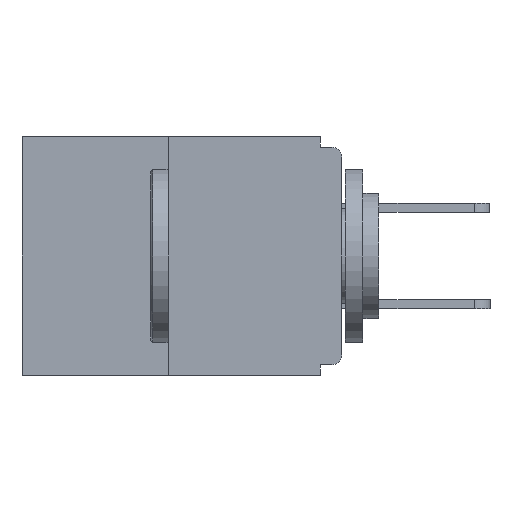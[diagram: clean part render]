
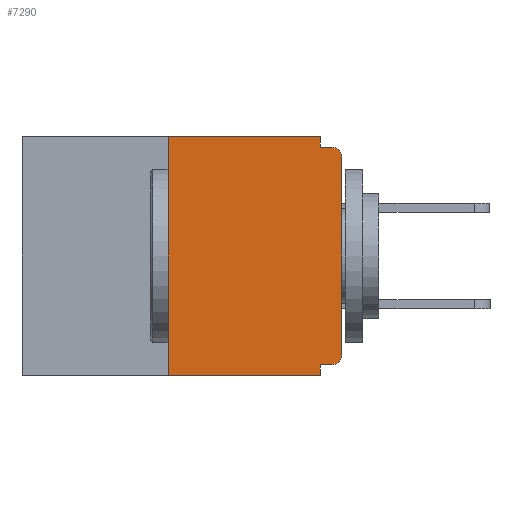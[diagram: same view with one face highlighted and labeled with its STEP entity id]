
A CAD part, left-side view. The second image highlights one B-rep face of the part: STEP entity #7290.
In plain terms, the highlighted planar face has unit normal (-1, 0, 0).
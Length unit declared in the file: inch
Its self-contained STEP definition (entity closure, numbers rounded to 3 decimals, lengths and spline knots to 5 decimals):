
#361 = DIRECTION ( 'NONE',  ( 1., 0., 0. ) ) ;
#381 = CARTESIAN_POINT ( 'NONE',  ( 0., 0.015, -0.03 ) ) ;
#546 = DIRECTION ( 'NONE',  ( 0., 0., -1. ) ) ;
#837 = CARTESIAN_POINT ( 'NONE',  ( 0., 0.25, 0. ) ) ;
#869 = CARTESIAN_POINT ( 'NONE',  ( 0., 0., 0. ) ) ;
#1276 = DIRECTION ( 'NONE',  ( 0., 0., -1. ) ) ;
#1318 = VECTOR ( 'NONE', #1604, 39.37008 ) ;
#1597 = CARTESIAN_POINT ( 'NONE',  ( 0., 0., -0.03 ) ) ;
#1604 = DIRECTION ( 'NONE',  ( 0., 0., -1. ) ) ;
#1741 = CARTESIAN_POINT ( 'NONE',  ( 0., 0., -0.313 ) ) ;
#1835 = CIRCLE ( 'NONE', #3360, 0.015 ) ;
#1837 = CARTESIAN_POINT ( 'NONE',  ( 0., 0.46, 0. ) ) ;
#1895 = CARTESIAN_POINT ( 'NONE',  ( 0., 0.25, 0. ) ) ;
#2158 = CARTESIAN_POINT ( 'NONE',  ( 0., 0.46, -0.343 ) ) ;
#2202 = LINE ( 'NONE', #4541, #16559 ) ;
#2294 = CARTESIAN_POINT ( 'NONE',  ( 0., 0., -0.328 ) ) ;
#2396 = ORIENTED_EDGE ( 'NONE', *, *, #13803, .T. ) ;
#2406 = DIRECTION ( 'NONE',  ( 0., 0., 1. ) ) ;
#3265 = VERTEX_POINT ( 'NONE', #7726 ) ;
#3360 = AXIS2_PLACEMENT_3D ( 'NONE', #381, #18469, #16746 ) ;
#4233 = ORIENTED_EDGE ( 'NONE', *, *, #10273, .T. ) ;
#4315 = CARTESIAN_POINT ( 'NONE',  ( 0., 0.031, -0.328 ) ) ;
#4493 = ORIENTED_EDGE ( 'NONE', *, *, #6026, .F. ) ;
#4526 = VERTEX_POINT ( 'NONE', #5584 ) ;
#4541 = CARTESIAN_POINT ( 'NONE',  ( 0., 0., -0.015 ) ) ;
#4764 = VERTEX_POINT ( 'NONE', #16749 ) ;
#5029 = ORIENTED_EDGE ( 'NONE', *, *, #14494, .F. ) ;
#5207 = EDGE_CURVE ( 'NONE', #5364, #18720, #5545, .T. ) ;
#5218 = ORIENTED_EDGE ( 'NONE', *, *, #16692, .F. ) ;
#5275 = VECTOR ( 'NONE', #16773, 39.37008 ) ;
#5364 = VERTEX_POINT ( 'NONE', #1741 ) ;
#5411 = VECTOR ( 'NONE', #18132, 39.37008 ) ;
#5515 = AXIS2_PLACEMENT_3D ( 'NONE', #13824, #361, #546 ) ;
#5545 = LINE ( 'NONE', #869, #19473 ) ;
#5584 = CARTESIAN_POINT ( 'NONE',  ( 0., 0.015, -0.015 ) ) ;
#5705 = ORIENTED_EDGE ( 'NONE', *, *, #17068, .F. ) ;
#5781 = LINE ( 'NONE', #8175, #14447 ) ;
#5806 = DIRECTION ( 'NONE',  ( -1., 0., 0. ) ) ;
#6026 = EDGE_CURVE ( 'NONE', #11294, #4526, #2202, .T. ) ;
#6120 = CARTESIAN_POINT ( 'NONE',  ( 0., 0.031, -0.343 ) ) ;
#6482 = PLANE ( 'NONE',  #5515 ) ;
#6616 = DIRECTION ( 'NONE',  ( 0., 0., -1. ) ) ;
#7290 = ADVANCED_FACE ( 'NONE', ( #10589 ), #6482, .F. ) ;
#7726 = CARTESIAN_POINT ( 'NONE',  ( 0., 0.031, -0.343 ) ) ;
#7785 = EDGE_CURVE ( 'NONE', #4764, #3265, #8707, .T. ) ;
#8097 = LINE ( 'NONE', #1837, #5275 ) ;
#8123 = CARTESIAN_POINT ( 'NONE',  ( 0., 0.031, -0.015 ) ) ;
#8175 = CARTESIAN_POINT ( 'NONE',  ( 0., 0.031, 0. ) ) ;
#8277 = EDGE_LOOP ( 'NONE', ( #5705, #5029, #16058, #8713, #19007, #4233, #8567, #2396, #4493, #5218 ) ) ;
#8366 = VECTOR ( 'NONE', #12908, 39.37008 ) ;
#8430 = VERTEX_POINT ( 'NONE', #4315 ) ;
#8567 = ORIENTED_EDGE ( 'NONE', *, *, #5207, .T. ) ;
#8707 = LINE ( 'NONE', #2158, #5411 ) ;
#8713 = ORIENTED_EDGE ( 'NONE', *, *, #19499, .F. ) ;
#9699 = VERTEX_POINT ( 'NONE', #18514 ) ;
#10273 = EDGE_CURVE ( 'NONE', #10338, #5364, #16638, .T. ) ;
#10338 = VERTEX_POINT ( 'NONE', #17808 ) ;
#10589 = FACE_OUTER_BOUND ( 'NONE', #8277, .T. ) ;
#10923 = AXIS2_PLACEMENT_3D ( 'NONE', #14912, #5806, #1276 ) ;
#11162 = LINE ( 'NONE', #2294, #8366 ) ;
#11294 = VERTEX_POINT ( 'NONE', #8123 ) ;
#11659 = LINE ( 'NONE', #6120, #1318 ) ;
#12330 = DIRECTION ( 'NONE',  ( 0., -1., 0. ) ) ;
#12908 = DIRECTION ( 'NONE',  ( 0., 1., 0. ) ) ;
#13803 = EDGE_CURVE ( 'NONE', #18720, #4526, #1835, .T. ) ;
#13824 = CARTESIAN_POINT ( 'NONE',  ( 0., 0.46, 0. ) ) ;
#14053 = LINE ( 'NONE', #837, #15000 ) ;
#14420 = VERTEX_POINT ( 'NONE', #1895 ) ;
#14447 = VECTOR ( 'NONE', #6616, 39.37008 ) ;
#14494 = EDGE_CURVE ( 'NONE', #4764, #14420, #14053, .T. ) ;
#14912 = CARTESIAN_POINT ( 'NONE',  ( 0., 0.015, -0.313 ) ) ;
#15000 = VECTOR ( 'NONE', #19092, 39.37008 ) ;
#15983 = EDGE_CURVE ( 'NONE', #10338, #8430, #11162, .T. ) ;
#16058 = ORIENTED_EDGE ( 'NONE', *, *, #7785, .T. ) ;
#16559 = VECTOR ( 'NONE', #12330, 39.37008 ) ;
#16638 = CIRCLE ( 'NONE', #10923, 0.015 ) ;
#16692 = EDGE_CURVE ( 'NONE', #9699, #11294, #5781, .T. ) ;
#16746 = DIRECTION ( 'NONE',  ( 0., 0., -1. ) ) ;
#16749 = CARTESIAN_POINT ( 'NONE',  ( 0., 0.25, -0.343 ) ) ;
#16773 = DIRECTION ( 'NONE',  ( 0., -1., 0. ) ) ;
#17068 = EDGE_CURVE ( 'NONE', #14420, #9699, #8097, .T. ) ;
#17808 = CARTESIAN_POINT ( 'NONE',  ( 0., 0.015, -0.328 ) ) ;
#18132 = DIRECTION ( 'NONE',  ( 0., -1., 0. ) ) ;
#18469 = DIRECTION ( 'NONE',  ( -1., 0., 0. ) ) ;
#18514 = CARTESIAN_POINT ( 'NONE',  ( 0., 0.031, 0. ) ) ;
#18720 = VERTEX_POINT ( 'NONE', #1597 ) ;
#19007 = ORIENTED_EDGE ( 'NONE', *, *, #15983, .F. ) ;
#19092 = DIRECTION ( 'NONE',  ( 0., 0., 1. ) ) ;
#19473 = VECTOR ( 'NONE', #2406, 39.37008 ) ;
#19499 = EDGE_CURVE ( 'NONE', #8430, #3265, #11659, .T. ) ;
